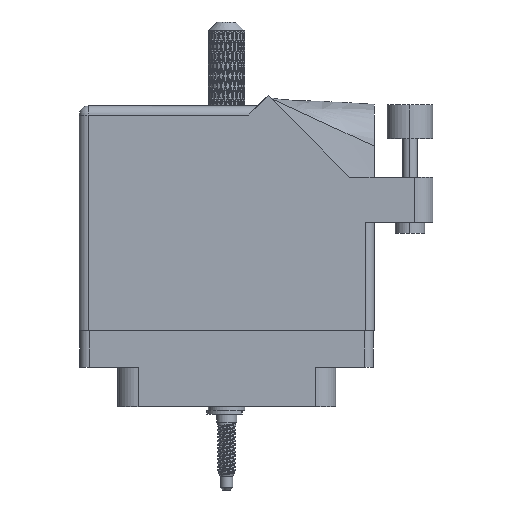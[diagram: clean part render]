
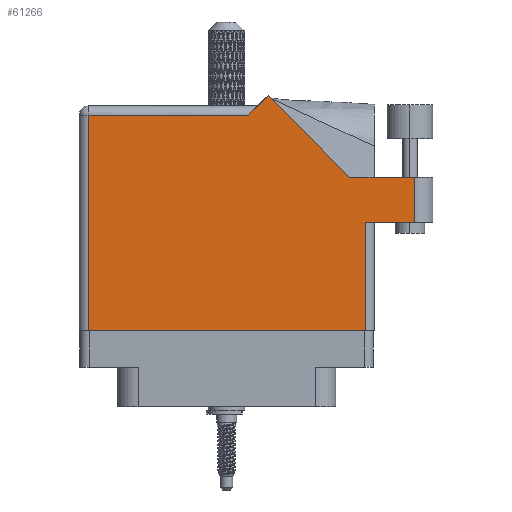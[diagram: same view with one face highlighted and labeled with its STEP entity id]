
A CAD part, front view. The second image highlights one B-rep face of the part: STEP entity #61266.
In plain terms, the highlighted face is planar.
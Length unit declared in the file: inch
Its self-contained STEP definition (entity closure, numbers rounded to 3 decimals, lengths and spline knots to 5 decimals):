
#929 = CARTESIAN_POINT ( 'NONE',  ( -0.943, -0.1, 0.455 ) ) ;
#971 = CARTESIAN_POINT ( 'NONE',  ( 1.28, 0.944, 0.455 ) ) ;
#4041 = VERTEX_POINT ( 'NONE', #43241 ) ;
#4583 = VECTOR ( 'NONE', #42665, 39.37008 ) ;
#6695 = VERTEX_POINT ( 'NONE', #79979 ) ;
#7832 = EDGE_CURVE ( 'NONE', #39719, #16241, #72124, .T. ) ;
#8029 = CARTESIAN_POINT ( 'NONE',  ( 1.005, 0.637, 0.455 ) ) ;
#8699 = CARTESIAN_POINT ( 'NONE',  ( 0.212, 1.43, 0.455 ) ) ;
#11433 = DIRECTION ( 'NONE',  ( 0., 0., -1. ) ) ;
#11612 = CARTESIAN_POINT ( 'NONE',  ( -1.005, 1.368, 0.455 ) ) ;
#11722 = EDGE_LOOP ( 'NONE', ( #64559, #98424, #72842, #56229, #37720, #23984, #74807, #51220, #99297 ) ) ;
#16241 = VERTEX_POINT ( 'NONE', #73844 ) ;
#16833 = EDGE_CURVE ( 'NONE', #94861, #6695, #56832, .T. ) ;
#18531 = VERTEX_POINT ( 'NONE', #103793 ) ;
#23394 = LINE ( 'NONE', #35547, #86043 ) ;
#23984 = ORIENTED_EDGE ( 'NONE', *, *, #74257, .T. ) ;
#25351 = DIRECTION ( 'NONE',  ( -0.707, -0.707, 0. ) ) ;
#28627 = CARTESIAN_POINT ( 'NONE',  ( 1.28, 0.944, 0.455 ) ) ;
#33824 = EDGE_CURVE ( 'NONE', #4041, #94861, #93324, .T. ) ;
#35547 = CARTESIAN_POINT ( 'NONE',  ( 1.405, 0.944, 0.455 ) ) ;
#37720 = ORIENTED_EDGE ( 'NONE', *, *, #7832, .T. ) ;
#38176 = CARTESIAN_POINT ( 'NONE',  ( -0.943, -0.1, 0.455 ) ) ;
#39719 = VERTEX_POINT ( 'NONE', #101105 ) ;
#41471 = VECTOR ( 'NONE', #80791, 39.37008 ) ;
#41620 = LINE ( 'NONE', #58764, #4583 ) ;
#42251 = CARTESIAN_POINT ( 'NONE',  ( 1.28, 0.637, 0.455 ) ) ;
#42665 = DIRECTION ( 'NONE',  ( -0.707, 0.707, 0. ) ) ;
#43241 = CARTESIAN_POINT ( 'NONE',  ( -0.943, 1.368, 0.455 ) ) ;
#46159 = DIRECTION ( 'NONE',  ( 0., 1., 0. ) ) ;
#50247 = LINE ( 'NONE', #95514, #93753 ) ;
#51220 = ORIENTED_EDGE ( 'NONE', *, *, #16833, .T. ) ;
#51253 = DIRECTION ( 'NONE',  ( -1., 0., 0. ) ) ;
#52879 = DIRECTION ( 'NONE',  ( -1., 0., 0. ) ) ;
#53260 = DIRECTION ( 'NONE',  ( 1., 0., 0. ) ) ;
#56229 = ORIENTED_EDGE ( 'NONE', *, *, #60880, .T. ) ;
#56832 = LINE ( 'NONE', #61555, #83722 ) ;
#58764 = CARTESIAN_POINT ( 'NONE',  ( 0.83942, 0.944, 0.455 ) ) ;
#60880 = EDGE_CURVE ( 'NONE', #18531, #39719, #41620, .T. ) ;
#61266 = ADVANCED_FACE ( 'NONE', ( #97821 ), #101762, .F. ) ;
#61555 = CARTESIAN_POINT ( 'NONE',  ( -1.005, -0.1, 0.455 ) ) ;
#64559 = ORIENTED_EDGE ( 'NONE', *, *, #96254, .T. ) ;
#66203 = LINE ( 'NONE', #971, #85339 ) ;
#72124 = LINE ( 'NONE', #8699, #88707 ) ;
#72842 = ORIENTED_EDGE ( 'NONE', *, *, #80778, .T. ) ;
#73844 = CARTESIAN_POINT ( 'NONE',  ( 0.15, 1.368, 0.455 ) ) ;
#74257 = EDGE_CURVE ( 'NONE', #16241, #4041, #102252, .T. ) ;
#74807 = ORIENTED_EDGE ( 'NONE', *, *, #33824, .T. ) ;
#75439 = VERTEX_POINT ( 'NONE', #88694 ) ;
#76049 = LINE ( 'NONE', #8029, #41471 ) ;
#76737 = DIRECTION ( 'NONE',  ( -1., 0., 0. ) ) ;
#79979 = CARTESIAN_POINT ( 'NONE',  ( 0.943, -0.1, 0.455 ) ) ;
#80393 = AXIS2_PLACEMENT_3D ( 'NONE', #100736, #11433, #76737 ) ;
#80778 = EDGE_CURVE ( 'NONE', #90763, #18531, #23394, .T. ) ;
#80791 = DIRECTION ( 'NONE',  ( 1., 0., 0. ) ) ;
#82716 = DIRECTION ( 'NONE',  ( 0., 1., 0. ) ) ;
#83722 = VECTOR ( 'NONE', #53260, 39.37008 ) ;
#85339 = VECTOR ( 'NONE', #82716, 39.37008 ) ;
#86043 = VECTOR ( 'NONE', #51253, 39.37008 ) ;
#88694 = CARTESIAN_POINT ( 'NONE',  ( 0.943, 0.637, 0.455 ) ) ;
#88707 = VECTOR ( 'NONE', #25351, 39.37008 ) ;
#90763 = VERTEX_POINT ( 'NONE', #28627 ) ;
#91675 = VERTEX_POINT ( 'NONE', #42251 ) ;
#93265 = EDGE_CURVE ( 'NONE', #91675, #90763, #66203, .T. ) ;
#93324 = LINE ( 'NONE', #38176, #98502 ) ;
#93753 = VECTOR ( 'NONE', #46159, 39.37008 ) ;
#94861 = VERTEX_POINT ( 'NONE', #929 ) ;
#95340 = DIRECTION ( 'NONE',  ( 0., -1., 0. ) ) ;
#95514 = CARTESIAN_POINT ( 'NONE',  ( 0.943, 0.637, 0.455 ) ) ;
#96254 = EDGE_CURVE ( 'NONE', #75439, #91675, #76049, .T. ) ;
#97028 = EDGE_CURVE ( 'NONE', #6695, #75439, #50247, .T. ) ;
#97821 = FACE_OUTER_BOUND ( 'NONE', #11722, .T. ) ;
#98424 = ORIENTED_EDGE ( 'NONE', *, *, #93265, .T. ) ;
#98483 = VECTOR ( 'NONE', #52879, 39.37008 ) ;
#98502 = VECTOR ( 'NONE', #95340, 39.37008 ) ;
#99297 = ORIENTED_EDGE ( 'NONE', *, *, #97028, .T. ) ;
#100736 = CARTESIAN_POINT ( 'NONE',  ( -1.005, 1.43, 0.455 ) ) ;
#101105 = CARTESIAN_POINT ( 'NONE',  ( 0.28271, 1.50071, 0.455 ) ) ;
#101762 = PLANE ( 'NONE',  #80393 ) ;
#102252 = LINE ( 'NONE', #11612, #98483 ) ;
#103793 = CARTESIAN_POINT ( 'NONE',  ( 0.83942, 0.944, 0.455 ) ) ;
